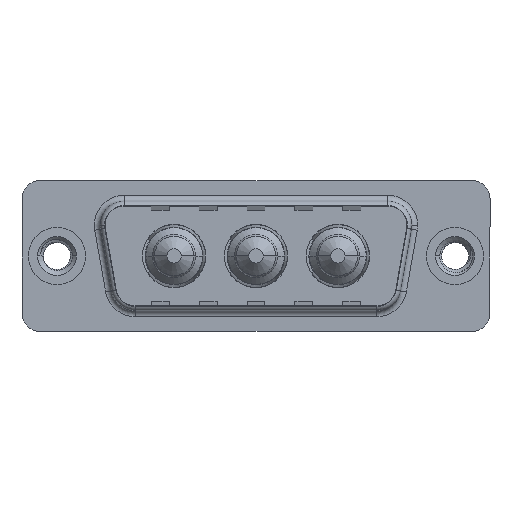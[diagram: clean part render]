
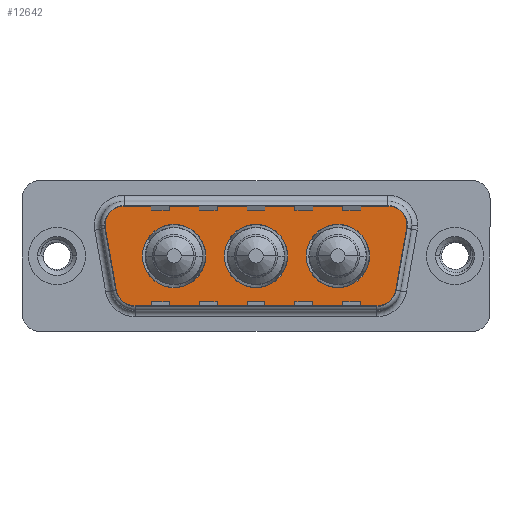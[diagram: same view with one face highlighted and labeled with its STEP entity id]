
A CAD part, top view. The second image highlights one B-rep face of the part: STEP entity #12642.
In plain terms, the highlighted planar face has unit normal (0, 0, 1).
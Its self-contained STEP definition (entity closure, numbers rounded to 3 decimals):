
#74 = CIRCLE ( 'NONE', #8440, 2. ) ;
#114 = ORIENTED_EDGE ( 'NONE', *, *, #866, .F. ) ;
#125 = EDGE_CURVE ( 'NONE', #164, #6111, #983, .T. ) ;
#164 = VERTEX_POINT ( 'NONE', #13480 ) ;
#283 = VERTEX_POINT ( 'NONE', #8161 ) ;
#325 = CARTESIAN_POINT ( 'NONE',  ( 5.411, 4.9, 0. ) ) ;
#416 = ORIENTED_EDGE ( 'NONE', *, *, #828, .F. ) ;
#613 = EDGE_CURVE ( 'NONE', #1030, #12044, #14782, .T. ) ;
#750 = AXIS2_PLACEMENT_3D ( 'NONE', #13071, #842, #9521 ) ;
#828 = EDGE_CURVE ( 'NONE', #13667, #12352, #6049, .T. ) ;
#842 = DIRECTION ( 'NONE',  ( 0., 0., 1. ) ) ;
#866 = EDGE_CURVE ( 'NONE', #6111, #164, #11800, .T. ) ;
#983 = CIRCLE ( 'NONE', #11275, 2.65 ) ;
#1021 = CARTESIAN_POINT ( 'NONE',  ( 26.866, -2.9, 0. ) ) ;
#1027 = EDGE_LOOP ( 'NONE', ( #4360, #416 ) ) ;
#1030 = VERTEX_POINT ( 'NONE', #2771 ) ;
#1074 = EDGE_CURVE ( 'NONE', #13896, #4763, #13062, .T. ) ;
#1226 = AXIS2_PLACEMENT_3D ( 'NONE', #15727, #1762, #6156 ) ;
#1353 = VECTOR ( 'NONE', #10430, 1000. ) ;
#1486 = DIRECTION ( 'NONE',  ( 0., 0., 1. ) ) ;
#1580 = VECTOR ( 'NONE', #13284, 1000. ) ;
#1627 = DIRECTION ( 'NONE',  ( 1., 0., 0. ) ) ;
#1760 = AXIS2_PLACEMENT_3D ( 'NONE', #11029, #4035, #2736 ) ;
#1762 = DIRECTION ( 'NONE',  ( 0., 0., 1. ) ) ;
#1809 = CARTESIAN_POINT ( 'NONE',  ( 9.8, 0., 0. ) ) ;
#1849 = CARTESIAN_POINT ( 'NONE',  ( 28.836, -3.247, 0. ) ) ;
#1886 = CARTESIAN_POINT ( 'NONE',  ( 29.859, 2.553, 0. ) ) ;
#1952 = CARTESIAN_POINT ( 'NONE',  ( 29.889, 2.9, 0. ) ) ;
#1989 = EDGE_CURVE ( 'NONE', #12352, #13667, #5633, .T. ) ;
#2081 = CARTESIAN_POINT ( 'NONE',  ( 4.464, -3.247, 0. ) ) ;
#2185 = ORIENTED_EDGE ( 'NONE', *, *, #7739, .T. ) ;
#2221 = ORIENTED_EDGE ( 'NONE', *, *, #14938, .T. ) ;
#2243 = CARTESIAN_POINT ( 'NONE',  ( 16.65, 0., 0. ) ) ;
#2260 = CIRCLE ( 'NONE', #6672, 2. ) ;
#2263 = DIRECTION ( 'NONE',  ( 1., 0., 0. ) ) ;
#2736 = DIRECTION ( 'NONE',  ( -1., 0., 0. ) ) ;
#2766 = DIRECTION ( 'NONE',  ( 0., 0., 1. ) ) ;
#2771 = CARTESIAN_POINT ( 'NONE',  ( 6.434, -4.9, 0. ) ) ;
#2826 = EDGE_CURVE ( 'NONE', #6899, #14776, #8374, .T. ) ;
#2895 = EDGE_CURVE ( 'NONE', #6487, #1030, #7227, .T. ) ;
#2948 = CARTESIAN_POINT ( 'NONE',  ( 27.889, 4.9, 0. ) ) ;
#3152 = ORIENTED_EDGE ( 'NONE', *, *, #1074, .F. ) ;
#3214 = DIRECTION ( 'NONE',  ( 0., 0., 1. ) ) ;
#3356 = EDGE_LOOP ( 'NONE', ( #9252, #11653, #2221, #5627, #11420, #6173, #2185, #7633, #15672 ) ) ;
#3445 = AXIS2_PLACEMENT_3D ( 'NONE', #1809, #8040, #15597 ) ;
#3610 = EDGE_LOOP ( 'NONE', ( #114, #13604 ) ) ;
#3738 = CARTESIAN_POINT ( 'NONE',  ( 26.866, -4.9, 0. ) ) ;
#3896 = CARTESIAN_POINT ( 'NONE',  ( 9.8, 0., 0. ) ) ;
#3955 = CIRCLE ( 'NONE', #13910, 2. ) ;
#4035 = DIRECTION ( 'NONE',  ( 0., 0., 1. ) ) ;
#4360 = ORIENTED_EDGE ( 'NONE', *, *, #1989, .F. ) ;
#4634 = FACE_BOUND ( 'NONE', #15261, .T. ) ;
#4763 = VERTEX_POINT ( 'NONE', #13477 ) ;
#4782 = EDGE_CURVE ( 'NONE', #5002, #5608, #10564, .T. ) ;
#5002 = VERTEX_POINT ( 'NONE', #1849 ) ;
#5024 = FACE_BOUND ( 'NONE', #1027, .T. ) ;
#5099 = AXIS2_PLACEMENT_3D ( 'NONE', #6793, #5683, #6664 ) ;
#5125 = DIRECTION ( 'NONE',  ( 1., 0., 0. ) ) ;
#5230 = DIRECTION ( 'NONE',  ( -1., 0., 0. ) ) ;
#5287 = CARTESIAN_POINT ( 'NONE',  ( 12.45, 0., 0. ) ) ;
#5315 = VERTEX_POINT ( 'NONE', #10234 ) ;
#5404 = AXIS2_PLACEMENT_3D ( 'NONE', #8042, #13556, #10803 ) ;
#5608 = VERTEX_POINT ( 'NONE', #1886 ) ;
#5627 = ORIENTED_EDGE ( 'NONE', *, *, #2826, .T. ) ;
#5633 = CIRCLE ( 'NONE', #5851, 2.65 ) ;
#5683 = DIRECTION ( 'NONE',  ( 0., 0., 1. ) ) ;
#5800 = PLANE ( 'NONE',  #750 ) ;
#5851 = AXIS2_PLACEMENT_3D ( 'NONE', #12113, #9766, #7220 ) ;
#5952 = VECTOR ( 'NONE', #5230, 1000. ) ;
#6049 = CIRCLE ( 'NONE', #1226, 2.65 ) ;
#6111 = VERTEX_POINT ( 'NONE', #8746 ) ;
#6156 = DIRECTION ( 'NONE',  ( 1., 0., 0. ) ) ;
#6173 = ORIENTED_EDGE ( 'NONE', *, *, #8487, .T. ) ;
#6239 = EDGE_CURVE ( 'NONE', #14776, #283, #12429, .T. ) ;
#6245 = CARTESIAN_POINT ( 'NONE',  ( 29.859, 2.553, 0. ) ) ;
#6487 = VERTEX_POINT ( 'NONE', #2081 ) ;
#6664 = DIRECTION ( 'NONE',  ( -1., 0., 0. ) ) ;
#6672 = AXIS2_PLACEMENT_3D ( 'NONE', #10607, #3214, #11832 ) ;
#6793 = CARTESIAN_POINT ( 'NONE',  ( 6.434, -2.9, 0. ) ) ;
#6899 = VERTEX_POINT ( 'NONE', #1952 ) ;
#7025 = EDGE_CURVE ( 'NONE', #12044, #5002, #3955, .T. ) ;
#7220 = DIRECTION ( 'NONE',  ( 1., 0., 0. ) ) ;
#7227 = CIRCLE ( 'NONE', #5099, 2. ) ;
#7360 = VECTOR ( 'NONE', #7535, 1000. ) ;
#7535 = DIRECTION ( 'NONE',  ( 0.174, 0.985, 0. ) ) ;
#7633 = ORIENTED_EDGE ( 'NONE', *, *, #2895, .T. ) ;
#7739 = EDGE_CURVE ( 'NONE', #5315, #6487, #8276, .T. ) ;
#8040 = DIRECTION ( 'NONE',  ( 0., 0., 1. ) ) ;
#8042 = CARTESIAN_POINT ( 'NONE',  ( 16.65, 0., 0. ) ) ;
#8161 = CARTESIAN_POINT ( 'NONE',  ( 5.411, 4.9, 0. ) ) ;
#8276 = LINE ( 'NONE', #12169, #1580 ) ;
#8374 = CIRCLE ( 'NONE', #1760, 2. ) ;
#8440 = AXIS2_PLACEMENT_3D ( 'NONE', #10176, #2766, #11404 ) ;
#8487 = EDGE_CURVE ( 'NONE', #283, #5315, #74, .T. ) ;
#8746 = CARTESIAN_POINT ( 'NONE',  ( 19.3, 0., 0. ) ) ;
#8762 = FACE_OUTER_BOUND ( 'NONE', #3356, .T. ) ;
#9252 = ORIENTED_EDGE ( 'NONE', *, *, #7025, .T. ) ;
#9521 = DIRECTION ( 'NONE',  ( 1., 0., 0. ) ) ;
#9619 = AXIS2_PLACEMENT_3D ( 'NONE', #3896, #12469, #5125 ) ;
#9700 = DIRECTION ( 'NONE',  ( 0., 0., 1. ) ) ;
#9766 = DIRECTION ( 'NONE',  ( 0., 0., 1. ) ) ;
#9945 = CARTESIAN_POINT ( 'NONE',  ( 20.85, 0., 0. ) ) ;
#10176 = CARTESIAN_POINT ( 'NONE',  ( 5.411, 2.9, 0. ) ) ;
#10234 = CARTESIAN_POINT ( 'NONE',  ( 3.441, 2.553, 0. ) ) ;
#10430 = DIRECTION ( 'NONE',  ( 1., 0., 0. ) ) ;
#10564 = LINE ( 'NONE', #6245, #7360 ) ;
#10607 = CARTESIAN_POINT ( 'NONE',  ( 27.889, 2.9, 0. ) ) ;
#10803 = DIRECTION ( 'NONE',  ( 1., 0., 0. ) ) ;
#11029 = CARTESIAN_POINT ( 'NONE',  ( 27.889, 2.9, 0. ) ) ;
#11275 = AXIS2_PLACEMENT_3D ( 'NONE', #2243, #1486, #1627 ) ;
#11404 = DIRECTION ( 'NONE',  ( 1., 0., 0. ) ) ;
#11420 = ORIENTED_EDGE ( 'NONE', *, *, #6239, .T. ) ;
#11653 = ORIENTED_EDGE ( 'NONE', *, *, #4782, .T. ) ;
#11800 = CIRCLE ( 'NONE', #5404, 2.65 ) ;
#11832 = DIRECTION ( 'NONE',  ( -1., 0., 0. ) ) ;
#12044 = VERTEX_POINT ( 'NONE', #3738 ) ;
#12113 = CARTESIAN_POINT ( 'NONE',  ( 23.5, 0., 0. ) ) ;
#12169 = CARTESIAN_POINT ( 'NONE',  ( 3.441, 2.553, 0. ) ) ;
#12352 = VERTEX_POINT ( 'NONE', #15183 ) ;
#12429 = LINE ( 'NONE', #325, #5952 ) ;
#12469 = DIRECTION ( 'NONE',  ( 0., 0., 1. ) ) ;
#12642 = ADVANCED_FACE ( 'NONE', ( #14373, #5024, #4634, #8762 ), #5800, .T. ) ;
#13062 = CIRCLE ( 'NONE', #3445, 2.65 ) ;
#13071 = CARTESIAN_POINT ( 'NONE',  ( 26.866, -2.9, 0. ) ) ;
#13284 = DIRECTION ( 'NONE',  ( 0.174, -0.985, 0. ) ) ;
#13477 = CARTESIAN_POINT ( 'NONE',  ( 7.15, 0., 0. ) ) ;
#13480 = CARTESIAN_POINT ( 'NONE',  ( 14., 0., 0. ) ) ;
#13556 = DIRECTION ( 'NONE',  ( 0., 0., 1. ) ) ;
#13604 = ORIENTED_EDGE ( 'NONE', *, *, #125, .F. ) ;
#13667 = VERTEX_POINT ( 'NONE', #9945 ) ;
#13896 = VERTEX_POINT ( 'NONE', #5287 ) ;
#13910 = AXIS2_PLACEMENT_3D ( 'NONE', #1021, #9700, #2263 ) ;
#14373 = FACE_BOUND ( 'NONE', #3610, .T. ) ;
#14492 = CARTESIAN_POINT ( 'NONE',  ( 6.434, -4.9, 0. ) ) ;
#14776 = VERTEX_POINT ( 'NONE', #2948 ) ;
#14782 = LINE ( 'NONE', #14492, #1353 ) ;
#14938 = EDGE_CURVE ( 'NONE', #5608, #6899, #2260, .T. ) ;
#15072 = CIRCLE ( 'NONE', #9619, 2.65 ) ;
#15183 = CARTESIAN_POINT ( 'NONE',  ( 26.15, 0., 0. ) ) ;
#15261 = EDGE_LOOP ( 'NONE', ( #3152, #15825 ) ) ;
#15335 = EDGE_CURVE ( 'NONE', #4763, #13896, #15072, .T. ) ;
#15597 = DIRECTION ( 'NONE',  ( 1., 0., 0. ) ) ;
#15672 = ORIENTED_EDGE ( 'NONE', *, *, #613, .T. ) ;
#15727 = CARTESIAN_POINT ( 'NONE',  ( 23.5, 0., 0. ) ) ;
#15825 = ORIENTED_EDGE ( 'NONE', *, *, #15335, .F. ) ;
